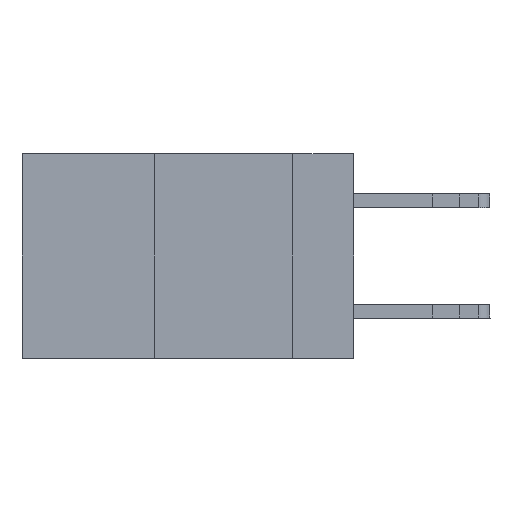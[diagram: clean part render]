
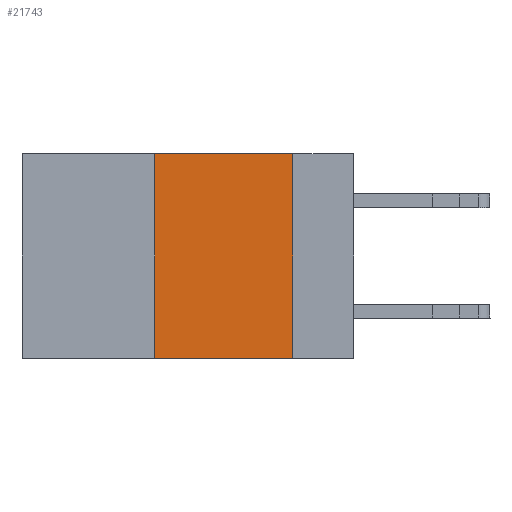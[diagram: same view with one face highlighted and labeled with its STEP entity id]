
A CAD part, left-side view. The second image highlights one B-rep face of the part: STEP entity #21743.
In plain terms, the highlighted planar face has unit normal (-1, 0, 0).
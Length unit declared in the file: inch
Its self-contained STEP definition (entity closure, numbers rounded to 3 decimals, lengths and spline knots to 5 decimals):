
#291 = DIRECTION ( 'NONE',  ( 0., -1., 0. ) ) ;
#1672 = DIRECTION ( 'NONE',  ( 1., 0., 0. ) ) ;
#1765 = DIRECTION ( 'NONE',  ( 0., 0., 1. ) ) ;
#2240 = DIRECTION ( 'NONE',  ( 0., -1., 0. ) ) ;
#2954 = VERTEX_POINT ( 'NONE', #5608 ) ;
#3545 = EDGE_LOOP ( 'NONE', ( #10397, #6308, #12487, #23193 ) ) ;
#3711 = FACE_OUTER_BOUND ( 'NONE', #3545, .T. ) ;
#4531 = DIRECTION ( 'NONE',  ( 0., 0., -1. ) ) ;
#4651 = CARTESIAN_POINT ( 'NONE',  ( 0., 0.11, 0. ) ) ;
#5608 = CARTESIAN_POINT ( 'NONE',  ( 0., 0.11, -0.37 ) ) ;
#5619 = PLANE ( 'NONE',  #11496 ) ;
#5959 = LINE ( 'NONE', #14095, #13776 ) ;
#6308 = ORIENTED_EDGE ( 'NONE', *, *, #23435, .F. ) ;
#6450 = LINE ( 'NONE', #4651, #9994 ) ;
#6745 = CARTESIAN_POINT ( 'NONE',  ( 0., 0.36, 0. ) ) ;
#9994 = VECTOR ( 'NONE', #4531, 39.37008 ) ;
#9996 = LINE ( 'NONE', #17765, #10760 ) ;
#10315 = CARTESIAN_POINT ( 'NONE',  ( 0., 0.36, -0.37 ) ) ;
#10397 = ORIENTED_EDGE ( 'NONE', *, *, #12002, .F. ) ;
#10456 = VERTEX_POINT ( 'NONE', #22250 ) ;
#10760 = VECTOR ( 'NONE', #291, 39.37008 ) ;
#11143 = EDGE_CURVE ( 'NONE', #18928, #15957, #14661, .T. ) ;
#11496 = AXIS2_PLACEMENT_3D ( 'NONE', #13029, #1672, #22748 ) ;
#12002 = EDGE_CURVE ( 'NONE', #10456, #2954, #6450, .T. ) ;
#12487 = ORIENTED_EDGE ( 'NONE', *, *, #11143, .F. ) ;
#13029 = CARTESIAN_POINT ( 'NONE',  ( 0., 0.6, 0. ) ) ;
#13776 = VECTOR ( 'NONE', #2240, 39.37008 ) ;
#14095 = CARTESIAN_POINT ( 'NONE',  ( 0., 0.6, -0.37 ) ) ;
#14661 = LINE ( 'NONE', #22476, #18184 ) ;
#14957 = EDGE_CURVE ( 'NONE', #18928, #2954, #5959, .T. ) ;
#15957 = VERTEX_POINT ( 'NONE', #6745 ) ;
#17765 = CARTESIAN_POINT ( 'NONE',  ( 0., 0.6, 0. ) ) ;
#18184 = VECTOR ( 'NONE', #1765, 39.37008 ) ;
#18928 = VERTEX_POINT ( 'NONE', #10315 ) ;
#21743 = ADVANCED_FACE ( 'NONE', ( #3711 ), #5619, .F. ) ;
#22250 = CARTESIAN_POINT ( 'NONE',  ( 0., 0.11, 0. ) ) ;
#22476 = CARTESIAN_POINT ( 'NONE',  ( 0., 0.36, 0. ) ) ;
#22748 = DIRECTION ( 'NONE',  ( 0., 0., -1. ) ) ;
#23193 = ORIENTED_EDGE ( 'NONE', *, *, #14957, .T. ) ;
#23435 = EDGE_CURVE ( 'NONE', #15957, #10456, #9996, .T. ) ;
